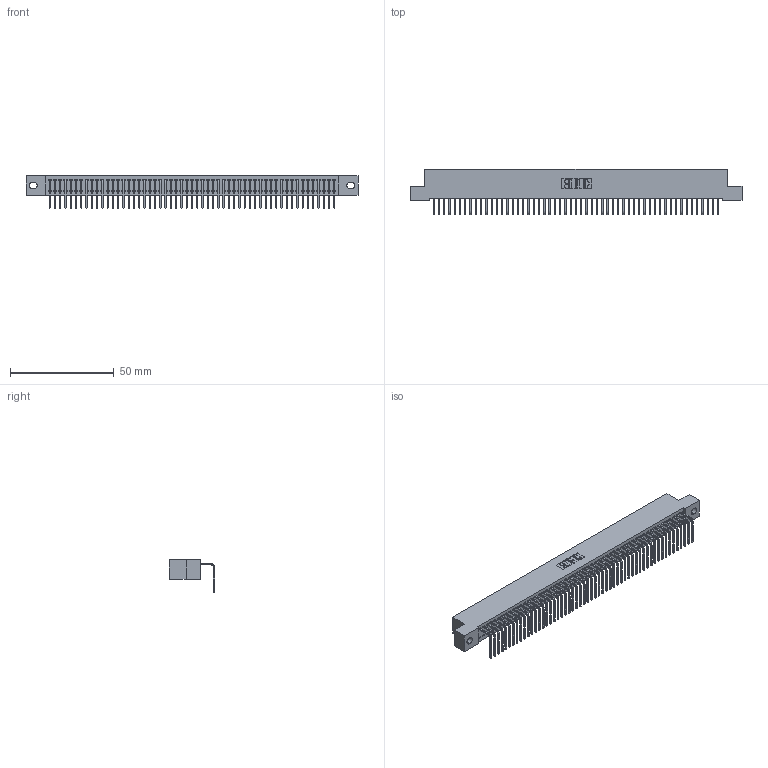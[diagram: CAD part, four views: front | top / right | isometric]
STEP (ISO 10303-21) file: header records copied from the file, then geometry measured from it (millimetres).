
FILE_DESCRIPTION (( 'STEP AP203' ), '1' );
FILE_NAME ('342-055-558-102.STEP', '2018-08-13T01:50:57', ( '' ), ( '' ), 'SwSTEP 2.0', 'SolidWorks 2016', '' );
FILE_SCHEMA (( 'CONFIG_CONTROL_DESIGN' ));
Length unit declared in the file: inch
Products named in the file (3): 342 Part_.128 Slot; 345-292-001_558 Tail - 2; 342-055-558-102
Assembly tree (56 placements, depth 2):
  342-055-558-102
    342 Part_.128 Slot
    345-292-001_558 Tail - 2  x55
Bounding box: 160.02 x 21.91 x 15.62 mm (x, y, z)
Volume: 14209.5 mm3; surface area: 21909.1 mm2
Topology: 56 solids, 56 shells, 3414 faces, 10321 edges, 6806 vertices
Faces by surface type: plane 2490, cylinder 924
Entity records: 32029 total; most frequent: CARTESIAN_POINT 5531, ORIENTED_EDGE 5522, DIRECTION 4639, EDGE_CURVE 2761, VECTOR 2633, LINE 2633, VERTEX_POINT 1838, AXIS2_PLACEMENT_3D 1003
